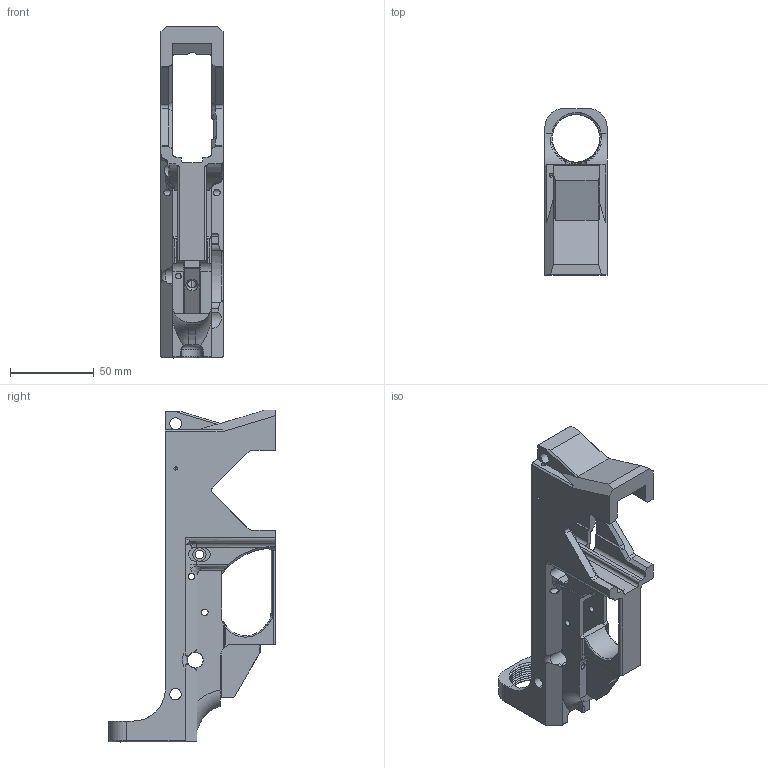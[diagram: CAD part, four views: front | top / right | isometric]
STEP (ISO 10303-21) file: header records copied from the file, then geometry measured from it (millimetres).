
FILE_DESCRIPTION((''),'2;1');
FILE_NAME('VANGUARD_AR15_V1_BY_SHADOWFALL','2014-02-26T',('Administrator'),(''),'PRO/ENGINEER BY PARAMETRIC TECHNOLOGY CORPORATION, 2012130','PRO/ENGINEER BY PARAMETRIC TECHNOLOGY CORPORATION, 2012130','');
FILE_SCHEMA(('CONFIG_CONTROL_DESIGN'));
Length unit declared in the file: millimetre
Products named in the file (1): VANGUARD_AR15_V1_BY_SHADOWFALL
Bounding box: 37.13 x 99.69 x 198.77 mm (x, y, z)
Volume: 153587.2 mm3; surface area: 56652.5 mm2
Topology: 1 solids, 1 shells, 508 faces, 1418 edges, 897 vertices
Faces by surface type: cylinder 208, plane 150, bspline 87, torus 42, cone 17, sphere 4
Entity records: 24658 total; most frequent: CARTESIAN_POINT 12324, ORIENTED_EDGE 2822, DIRECTION 2247, EDGE_CURVE 1411, VERTEX_POINT 897, AXIS2_PLACEMENT_3D 807, VECTOR 633, LINE 633
